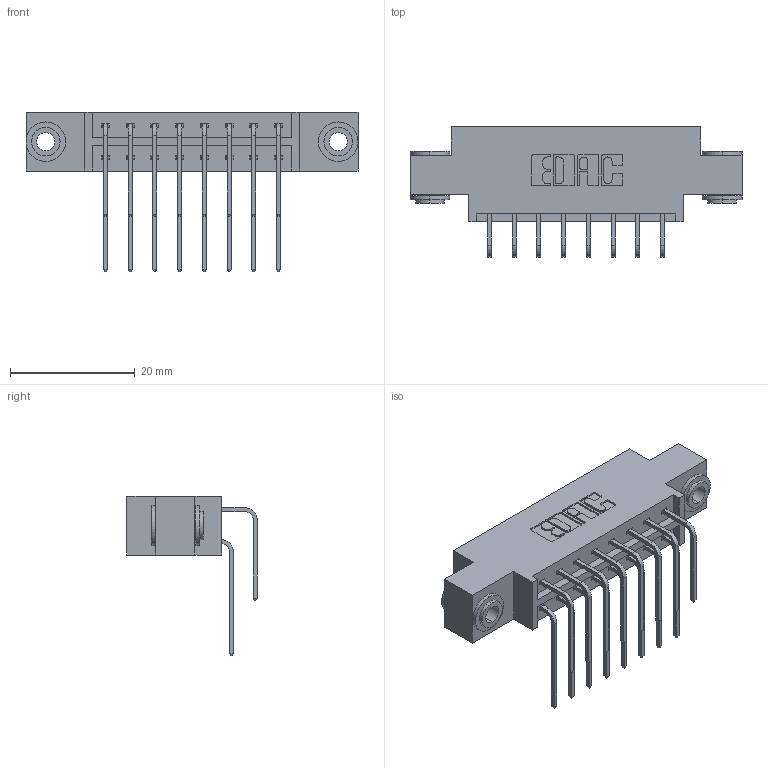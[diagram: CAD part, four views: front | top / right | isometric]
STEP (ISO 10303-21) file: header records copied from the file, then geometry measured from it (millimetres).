
FILE_DESCRIPTION (( 'STEP AP203' ), '1' );
FILE_NAME ('833-016-559-803.STEP', '2020-05-31T19:15:18', ( '' ), ( '' ), 'SwSTEP 2.0', 'SolidWorks 2020', '' );
FILE_SCHEMA (( 'CONFIG_CONTROL_DESIGN' ));
Length unit declared in the file: inch
Products named in the file (5): 345-250-002_345-250-002-102; 345-292-001_558 559 Tail - 1; 345-292-001_559 Tail - 2; 833 Part_Offset - .156 Dia - TH; 833-016-559-803
Assembly tree (19 placements, depth 2):
  833-016-559-803
    833 Part_Offset - .156 Dia - TH
    345-292-001_558 559 Tail - 1  x8
    345-292-001_559 Tail - 2  x8
    345-250-002_345-250-002-102  x2
Bounding box: 53.24 x 20.9 x 25.53 mm (x, y, z)
Volume: 5001.3 mm3; surface area: 6448.9 mm2
Topology: 19 solids, 19 shells, 1020 faces, 2975 edges, 1958 vertices
Faces by surface type: plane 692, cylinder 320, cone 8
Entity records: 12110 total; most frequent: CARTESIAN_POINT 2076, ORIENTED_EDGE 1954, DIRECTION 1847, EDGE_CURVE 977, LINE 785, VECTOR 785, VERTEX_POINT 646, AXIS2_PLACEMENT_3D 531
